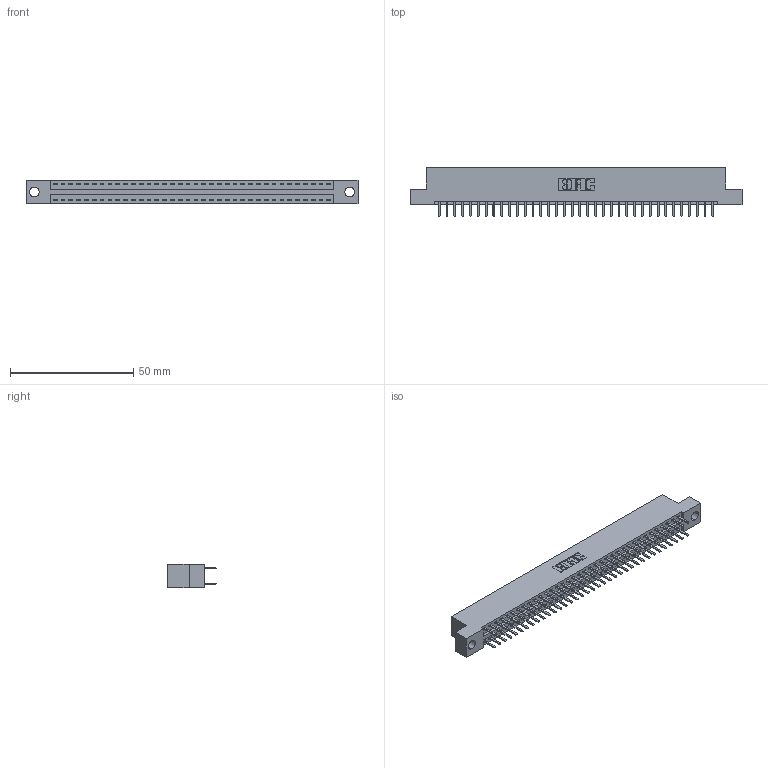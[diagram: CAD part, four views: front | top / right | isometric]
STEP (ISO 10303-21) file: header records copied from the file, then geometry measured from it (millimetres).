
FILE_DESCRIPTION (( 'STEP AP203' ), '1' );
FILE_NAME ('346-072-520-204.STEP', '2022-05-24T23:05:27', ( '' ), ( '' ), 'SwSTEP 2.0', 'SolidWorks 2020', '' );
FILE_SCHEMA (( 'CONFIG_CONTROL_DESIGN' ));
Length unit declared in the file: inch
Products named in the file (3): 345-292-001_345-293-120; 346-072-520-204; 346 Part_Flush Mounting Lugs - 0.156 Dia-TH
Assembly tree (73 placements, depth 2):
  346-072-520-204
    346 Part_Flush Mounting Lugs - 0.156 Dia-TH
    345-292-001_345-293-120  x72
Bounding box: 134.87 x 20.02 x 9.4 mm (x, y, z)
Volume: 12967.7 mm3; surface area: 17504.4 mm2
Topology: 73 solids, 73 shells, 4168 faces, 12101 edges, 7874 vertices
Faces by surface type: plane 2754, cylinder 1414
Entity records: 24835 total; most frequent: CARTESIAN_POINT 4118, ORIENTED_EDGE 4038, DIRECTION 3667, EDGE_CURVE 2019, VECTOR 1739, LINE 1739, VERTEX_POINT 1342, AXIS2_PLACEMENT_3D 964
